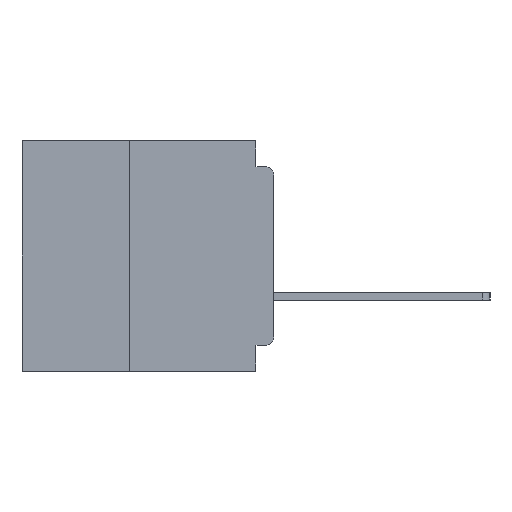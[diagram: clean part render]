
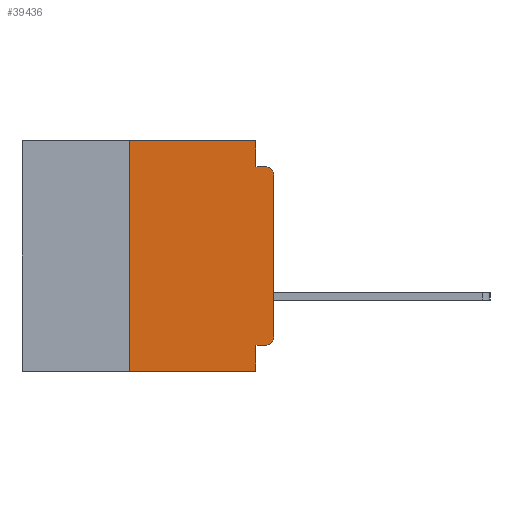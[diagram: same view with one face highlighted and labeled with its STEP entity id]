
A CAD part, left-side view. The second image highlights one B-rep face of the part: STEP entity #39436.
In plain terms, the highlighted planar face has unit normal (-1, 0, 0).
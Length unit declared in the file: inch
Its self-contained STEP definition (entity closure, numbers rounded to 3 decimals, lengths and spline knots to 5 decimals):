
#189 = ORIENTED_EDGE ( 'NONE', *, *, #40179, .F. ) ;
#1586 = FACE_OUTER_BOUND ( 'NONE', #6209, .T. ) ;
#1733 = DIRECTION ( 'NONE',  ( 0., 0., 1. ) ) ;
#1767 = CARTESIAN_POINT ( 'NONE',  ( 0., 0., -0.355 ) ) ;
#2032 = VERTEX_POINT ( 'NONE', #36778 ) ;
#2295 = EDGE_CURVE ( 'NONE', #30179, #38848, #41159, .T. ) ;
#2403 = CARTESIAN_POINT ( 'NONE',  ( 0., 0.437, -0.4 ) ) ;
#2815 = ORIENTED_EDGE ( 'NONE', *, *, #39226, .T. ) ;
#4160 = DIRECTION ( 'NONE',  ( -1., 0., 0. ) ) ;
#4439 = CARTESIAN_POINT ( 'NONE',  ( 0., 0.031, -0.045 ) ) ;
#5411 = ORIENTED_EDGE ( 'NONE', *, *, #2295, .F. ) ;
#5737 = DIRECTION ( 'NONE',  ( 0., -1., 0. ) ) ;
#6092 = CARTESIAN_POINT ( 'NONE',  ( 0., 0., -0.06 ) ) ;
#6209 = EDGE_LOOP ( 'NONE', ( #2815, #12779, #18665, #5411, #189, #29036, #29375, #30087, #16146, #10713 ) ) ;
#6259 = VECTOR ( 'NONE', #5737, 39.37008 ) ;
#6702 = LINE ( 'NONE', #31223, #38048 ) ;
#6897 = AXIS2_PLACEMENT_3D ( 'NONE', #40071, #7595, #30572 ) ;
#7319 = LINE ( 'NONE', #2403, #6259 ) ;
#7459 = CARTESIAN_POINT ( 'NONE',  ( 0., 0.015, -0.355 ) ) ;
#7595 = DIRECTION ( 'NONE',  ( 1., 0., 0. ) ) ;
#7823 = LINE ( 'NONE', #17093, #32949 ) ;
#7850 = VECTOR ( 'NONE', #9786, 39.37008 ) ;
#8292 = DIRECTION ( 'NONE',  ( 0., 1., 0. ) ) ;
#9369 = CARTESIAN_POINT ( 'NONE',  ( 0., 0.031, -0.4 ) ) ;
#9786 = DIRECTION ( 'NONE',  ( 0., 0., 1. ) ) ;
#10157 = AXIS2_PLACEMENT_3D ( 'NONE', #23925, #4160, #27179 ) ;
#10713 = ORIENTED_EDGE ( 'NONE', *, *, #29043, .T. ) ;
#10814 = PLANE ( 'NONE',  #6897 ) ;
#12114 = VECTOR ( 'NONE', #35418, 39.37008 ) ;
#12497 = EDGE_CURVE ( 'NONE', #28112, #34556, #37183, .T. ) ;
#12534 = CARTESIAN_POINT ( 'NONE',  ( 0., 0.031, -0.4 ) ) ;
#12564 = VERTEX_POINT ( 'NONE', #19139 ) ;
#12779 = ORIENTED_EDGE ( 'NONE', *, *, #36018, .T. ) ;
#14092 = VERTEX_POINT ( 'NONE', #7459 ) ;
#15856 = EDGE_CURVE ( 'NONE', #38848, #2032, #7823, .T. ) ;
#16146 = ORIENTED_EDGE ( 'NONE', *, *, #17549, .F. ) ;
#17093 = CARTESIAN_POINT ( 'NONE',  ( 0., 0., -0.045 ) ) ;
#17433 = CARTESIAN_POINT ( 'NONE',  ( 0., 0.015, -0.34 ) ) ;
#17549 = EDGE_CURVE ( 'NONE', #14092, #28112, #35882, .T. ) ;
#18665 = ORIENTED_EDGE ( 'NONE', *, *, #15856, .F. ) ;
#19139 = CARTESIAN_POINT ( 'NONE',  ( 0., 0.25, -0.4 ) ) ;
#20362 = DIRECTION ( 'NONE',  ( 0., -1., 0. ) ) ;
#20688 = DIRECTION ( 'NONE',  ( 0., 0., -1. ) ) ;
#22208 = VECTOR ( 'NONE', #22930, 39.37008 ) ;
#22254 = EDGE_CURVE ( 'NONE', #12564, #31238, #6702, .T. ) ;
#22921 = CARTESIAN_POINT ( 'NONE',  ( 0., 0.031, 0. ) ) ;
#22930 = DIRECTION ( 'NONE',  ( 0., -1., 0. ) ) ;
#23037 = VERTEX_POINT ( 'NONE', #6092 ) ;
#23925 = CARTESIAN_POINT ( 'NONE',  ( 0., 0.015, -0.06 ) ) ;
#24017 = AXIS2_PLACEMENT_3D ( 'NONE', #17433, #40204, #20688 ) ;
#25591 = CARTESIAN_POINT ( 'NONE',  ( 0., 0.25, 0. ) ) ;
#27179 = DIRECTION ( 'NONE',  ( 0., 0., -1. ) ) ;
#27182 = VECTOR ( 'NONE', #8292, 39.37008 ) ;
#27870 = DIRECTION ( 'NONE',  ( 0., 0., -1. ) ) ;
#28062 = CARTESIAN_POINT ( 'NONE',  ( 0., 0.031, -0.355 ) ) ;
#28112 = VERTEX_POINT ( 'NONE', #28062 ) ;
#29036 = ORIENTED_EDGE ( 'NONE', *, *, #22254, .F. ) ;
#29043 = EDGE_CURVE ( 'NONE', #14092, #29511, #36994, .T. ) ;
#29191 = CARTESIAN_POINT ( 'NONE',  ( 0., 0.437, 0. ) ) ;
#29375 = ORIENTED_EDGE ( 'NONE', *, *, #32960, .T. ) ;
#29439 = CARTESIAN_POINT ( 'NONE',  ( 0., 0., 0. ) ) ;
#29511 = VERTEX_POINT ( 'NONE', #35800 ) ;
#30087 = ORIENTED_EDGE ( 'NONE', *, *, #12497, .F. ) ;
#30179 = VERTEX_POINT ( 'NONE', #22921 ) ;
#30572 = DIRECTION ( 'NONE',  ( 0., 0., -1. ) ) ;
#31223 = CARTESIAN_POINT ( 'NONE',  ( 0., 0.25, -0.4 ) ) ;
#31238 = VERTEX_POINT ( 'NONE', #25591 ) ;
#32089 = CARTESIAN_POINT ( 'NONE',  ( 0., 0.031, 0. ) ) ;
#32506 = VECTOR ( 'NONE', #27870, 39.37008 ) ;
#32886 = LINE ( 'NONE', #29191, #22208 ) ;
#32949 = VECTOR ( 'NONE', #20362, 39.37008 ) ;
#32960 = EDGE_CURVE ( 'NONE', #12564, #34556, #7319, .T. ) ;
#34556 = VERTEX_POINT ( 'NONE', #9369 ) ;
#35418 = DIRECTION ( 'NONE',  ( 0., 0., -1. ) ) ;
#35800 = CARTESIAN_POINT ( 'NONE',  ( 0., 0., -0.34 ) ) ;
#35882 = LINE ( 'NONE', #1767, #27182 ) ;
#36018 = EDGE_CURVE ( 'NONE', #23037, #2032, #41411, .T. ) ;
#36778 = CARTESIAN_POINT ( 'NONE',  ( 0., 0.015, -0.045 ) ) ;
#36994 = CIRCLE ( 'NONE', #24017, 0.015 ) ;
#37183 = LINE ( 'NONE', #12534, #12114 ) ;
#38048 = VECTOR ( 'NONE', #1733, 39.37008 ) ;
#38848 = VERTEX_POINT ( 'NONE', #4439 ) ;
#39226 = EDGE_CURVE ( 'NONE', #29511, #23037, #41643, .T. ) ;
#39436 = ADVANCED_FACE ( 'NONE', ( #1586 ), #10814, .F. ) ;
#40071 = CARTESIAN_POINT ( 'NONE',  ( 0., 0.437, 0. ) ) ;
#40179 = EDGE_CURVE ( 'NONE', #31238, #30179, #32886, .T. ) ;
#40204 = DIRECTION ( 'NONE',  ( -1., 0., 0. ) ) ;
#41159 = LINE ( 'NONE', #32089, #32506 ) ;
#41411 = CIRCLE ( 'NONE', #10157, 0.015 ) ;
#41643 = LINE ( 'NONE', #29439, #7850 ) ;
